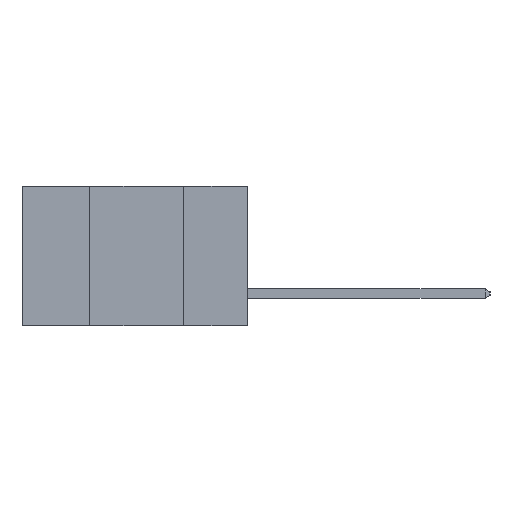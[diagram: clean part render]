
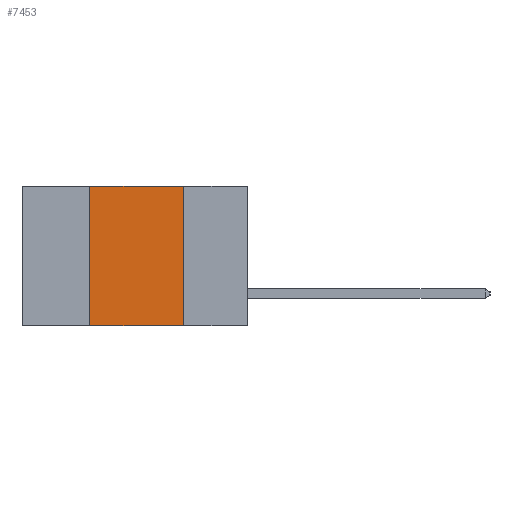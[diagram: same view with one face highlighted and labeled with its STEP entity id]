
A CAD part, left-side view. The second image highlights one B-rep face of the part: STEP entity #7453.
In plain terms, the highlighted planar face has unit normal (-1, 0, 0).
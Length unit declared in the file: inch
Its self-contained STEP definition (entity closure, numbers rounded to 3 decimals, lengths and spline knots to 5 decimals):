
#193 = LINE ( 'NONE', #13074, #11068 ) ;
#328 = CARTESIAN_POINT ( 'NONE',  ( 0., 0.6, 0. ) ) ;
#396 = VECTOR ( 'NONE', #13424, 39.37008 ) ;
#413 = AXIS2_PLACEMENT_3D ( 'NONE', #11972, #6894, #517 ) ;
#517 = DIRECTION ( 'NONE',  ( 0., 0., -1. ) ) ;
#2020 = VERTEX_POINT ( 'NONE', #9710 ) ;
#2214 = LINE ( 'NONE', #10139, #13266 ) ;
#2435 = VECTOR ( 'NONE', #7789, 39.37008 ) ;
#2873 = ORIENTED_EDGE ( 'NONE', *, *, #8934, .F. ) ;
#2942 = ORIENTED_EDGE ( 'NONE', *, *, #11639, .F. ) ;
#3010 = ORIENTED_EDGE ( 'NONE', *, *, #10292, .F. ) ;
#3054 = ORIENTED_EDGE ( 'NONE', *, *, #9607, .T. ) ;
#4784 = PLANE ( 'NONE',  #413 ) ;
#6591 = EDGE_LOOP ( 'NONE', ( #2873, #2942, #3010, #3054 ) ) ;
#6894 = DIRECTION ( 'NONE',  ( 1., 0., 0. ) ) ;
#7322 = CARTESIAN_POINT ( 'NONE',  ( 0., 0.17, -0.37 ) ) ;
#7453 = ADVANCED_FACE ( 'NONE', ( #7462 ), #4784, .F. ) ;
#7462 = FACE_OUTER_BOUND ( 'NONE', #6591, .T. ) ;
#7597 = CARTESIAN_POINT ( 'NONE',  ( 0., 0.42, -0.37 ) ) ;
#7789 = DIRECTION ( 'NONE',  ( 0., -1., 0. ) ) ;
#8934 = EDGE_CURVE ( 'NONE', #13506, #12646, #11557, .T. ) ;
#9057 = DIRECTION ( 'NONE',  ( 0., -1., 0. ) ) ;
#9106 = VERTEX_POINT ( 'NONE', #7597 ) ;
#9607 = EDGE_CURVE ( 'NONE', #9106, #12646, #193, .T. ) ;
#9710 = CARTESIAN_POINT ( 'NONE',  ( 0., 0.42, 0. ) ) ;
#10139 = CARTESIAN_POINT ( 'NONE',  ( 0., 0.42, -0.37 ) ) ;
#10292 = EDGE_CURVE ( 'NONE', #9106, #2020, #2214, .T. ) ;
#11068 = VECTOR ( 'NONE', #9057, 39.37008 ) ;
#11557 = LINE ( 'NONE', #7322, #396 ) ;
#11639 = EDGE_CURVE ( 'NONE', #2020, #13506, #12847, .T. ) ;
#11699 = CARTESIAN_POINT ( 'NONE',  ( 0., 0.17, 0. ) ) ;
#11972 = CARTESIAN_POINT ( 'NONE',  ( 0., 0.6, 0. ) ) ;
#12404 = CARTESIAN_POINT ( 'NONE',  ( 0., 0.17, -0.37 ) ) ;
#12646 = VERTEX_POINT ( 'NONE', #12404 ) ;
#12847 = LINE ( 'NONE', #328, #2435 ) ;
#13074 = CARTESIAN_POINT ( 'NONE',  ( 0., 0.6, -0.37 ) ) ;
#13147 = DIRECTION ( 'NONE',  ( 0., 0., 1. ) ) ;
#13266 = VECTOR ( 'NONE', #13147, 39.37008 ) ;
#13424 = DIRECTION ( 'NONE',  ( 0., 0., -1. ) ) ;
#13506 = VERTEX_POINT ( 'NONE', #11699 ) ;
